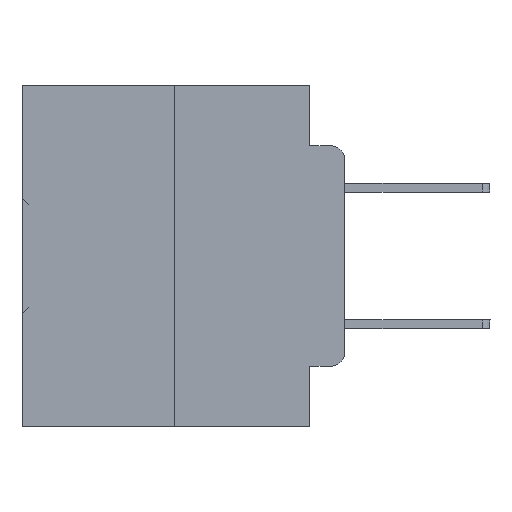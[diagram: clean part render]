
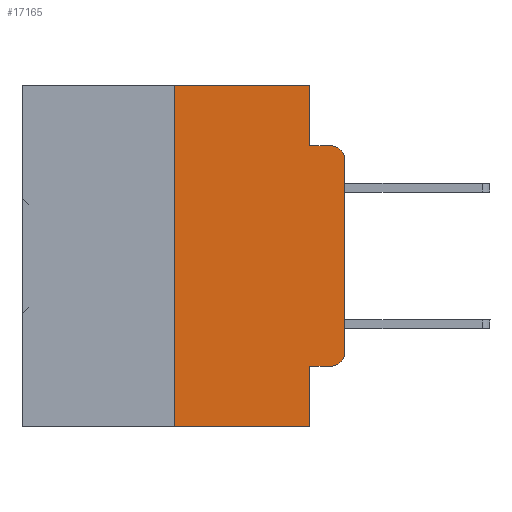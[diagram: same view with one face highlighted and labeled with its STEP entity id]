
A CAD part, left-side view. The second image highlights one B-rep face of the part: STEP entity #17165.
In plain terms, the highlighted planar face has unit normal (-1, 0, 0).
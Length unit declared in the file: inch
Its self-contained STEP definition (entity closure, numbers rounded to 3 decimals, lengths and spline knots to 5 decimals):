
#58 = EDGE_CURVE ( 'NONE', #10049, #34746, #6923, .T. ) ;
#234 = ORIENTED_EDGE ( 'NONE', *, *, #13687, .T. ) ;
#390 = CARTESIAN_POINT ( 'NONE',  ( 0., 0.473, 0. ) ) ;
#2044 = EDGE_LOOP ( 'NONE', ( #27411, #15511, #11126, #6072, #4916, #24331, #11601, #9806, #234, #10840 ) ) ;
#2606 = DIRECTION ( 'NONE',  ( 0., -1., 0. ) ) ;
#2704 = CARTESIAN_POINT ( 'NONE',  ( 0., 0.02, -0.4115 ) ) ;
#3750 = VECTOR ( 'NONE', #23329, 39.37008 ) ;
#4247 = DIRECTION ( 'NONE',  ( 0., 0., 1. ) ) ;
#4435 = EDGE_CURVE ( 'NONE', #4634, #13267, #22288, .T. ) ;
#4634 = VERTEX_POINT ( 'NONE', #22484 ) ;
#4916 = ORIENTED_EDGE ( 'NONE', *, *, #29884, .F. ) ;
#6008 = CARTESIAN_POINT ( 'NONE',  ( 0., 0.02, -0.0885 ) ) ;
#6072 = ORIENTED_EDGE ( 'NONE', *, *, #36249, .F. ) ;
#6174 = AXIS2_PLACEMENT_3D ( 'NONE', #25343, #8117, #22638 ) ;
#6923 = LINE ( 'NONE', #33304, #32812 ) ;
#8117 = DIRECTION ( 'NONE',  ( 1., 0., 0. ) ) ;
#8568 = DIRECTION ( 'NONE',  ( -1., 0., 0. ) ) ;
#8972 = DIRECTION ( 'NONE',  ( 0., 0., -1. ) ) ;
#9005 = LINE ( 'NONE', #390, #3750 ) ;
#9806 = ORIENTED_EDGE ( 'NONE', *, *, #4435, .F. ) ;
#9873 = DIRECTION ( 'NONE',  ( 0., 0., 1. ) ) ;
#10049 = VERTEX_POINT ( 'NONE', #32970 ) ;
#10840 = ORIENTED_EDGE ( 'NONE', *, *, #20039, .T. ) ;
#11126 = ORIENTED_EDGE ( 'NONE', *, *, #16709, .F. ) ;
#11536 = EDGE_CURVE ( 'NONE', #12909, #25795, #29789, .T. ) ;
#11601 = ORIENTED_EDGE ( 'NONE', *, *, #18489, .T. ) ;
#11685 = CARTESIAN_POINT ( 'NONE',  ( 0., 0.051, -0.5 ) ) ;
#11853 = CARTESIAN_POINT ( 'NONE',  ( 0., 0., -0.1085 ) ) ;
#12909 = VERTEX_POINT ( 'NONE', #31852 ) ;
#12980 = VECTOR ( 'NONE', #27152, 39.37008 ) ;
#13267 = VERTEX_POINT ( 'NONE', #11685 ) ;
#13687 = EDGE_CURVE ( 'NONE', #4634, #21027, #20557, .T. ) ;
#14054 = PLANE ( 'NONE',  #6174 ) ;
#15105 = CARTESIAN_POINT ( 'NONE',  ( 0., 0.473, -0.5 ) ) ;
#15511 = ORIENTED_EDGE ( 'NONE', *, *, #16609, .T. ) ;
#16229 = VECTOR ( 'NONE', #8972, 39.37008 ) ;
#16367 = DIRECTION ( 'NONE',  ( 0., 0., -1. ) ) ;
#16609 = EDGE_CURVE ( 'NONE', #25795, #22308, #25700, .T. ) ;
#16709 = EDGE_CURVE ( 'NONE', #36345, #22308, #19630, .T. ) ;
#17165 = ADVANCED_FACE ( 'NONE', ( #25149 ), #14054, .F. ) ;
#17486 = VECTOR ( 'NONE', #2606, 39.37008 ) ;
#18134 = CARTESIAN_POINT ( 'NONE',  ( 0., 0.051, 0. ) ) ;
#18489 = EDGE_CURVE ( 'NONE', #10049, #13267, #21007, .T. ) ;
#18982 = AXIS2_PLACEMENT_3D ( 'NONE', #33803, #24819, #36470 ) ;
#19630 = LINE ( 'NONE', #22310, #29960 ) ;
#19846 = CARTESIAN_POINT ( 'NONE',  ( 0., 0.25, 0. ) ) ;
#20039 = EDGE_CURVE ( 'NONE', #21027, #12909, #23960, .T. ) ;
#20339 = VERTEX_POINT ( 'NONE', #30192 ) ;
#20557 = LINE ( 'NONE', #28794, #17486 ) ;
#21007 = LINE ( 'NONE', #15105, #12980 ) ;
#21027 = VERTEX_POINT ( 'NONE', #2704 ) ;
#21909 = CARTESIAN_POINT ( 'NONE',  ( 0., 0.051, 0. ) ) ;
#22288 = LINE ( 'NONE', #21909, #33633 ) ;
#22308 = VERTEX_POINT ( 'NONE', #6008 ) ;
#22310 = CARTESIAN_POINT ( 'NONE',  ( 0., 0.051, -0.0885 ) ) ;
#22484 = CARTESIAN_POINT ( 'NONE',  ( 0., 0.051, -0.4115 ) ) ;
#22638 = DIRECTION ( 'NONE',  ( 0., 0., -1. ) ) ;
#23329 = DIRECTION ( 'NONE',  ( 0., -1., 0. ) ) ;
#23960 = CIRCLE ( 'NONE', #26433, 0.02 ) ;
#24331 = ORIENTED_EDGE ( 'NONE', *, *, #58, .F. ) ;
#24598 = CARTESIAN_POINT ( 'NONE',  ( 0., 0., 0. ) ) ;
#24819 = DIRECTION ( 'NONE',  ( -1., 0., 0. ) ) ;
#25149 = FACE_OUTER_BOUND ( 'NONE', #2044, .T. ) ;
#25343 = CARTESIAN_POINT ( 'NONE',  ( 0., 0.473, 0. ) ) ;
#25584 = DIRECTION ( 'NONE',  ( 0., -1., 0. ) ) ;
#25700 = CIRCLE ( 'NONE', #18982, 0.02 ) ;
#25795 = VERTEX_POINT ( 'NONE', #11853 ) ;
#26358 = CARTESIAN_POINT ( 'NONE',  ( 0., 0.02, -0.3915 ) ) ;
#26433 = AXIS2_PLACEMENT_3D ( 'NONE', #26358, #8568, #32297 ) ;
#27152 = DIRECTION ( 'NONE',  ( 0., -1., 0. ) ) ;
#27411 = ORIENTED_EDGE ( 'NONE', *, *, #11536, .T. ) ;
#28461 = VECTOR ( 'NONE', #9873, 39.37008 ) ;
#28794 = CARTESIAN_POINT ( 'NONE',  ( 0., 0.051, -0.4115 ) ) ;
#29789 = LINE ( 'NONE', #24598, #28461 ) ;
#29884 = EDGE_CURVE ( 'NONE', #34746, #20339, #9005, .T. ) ;
#29960 = VECTOR ( 'NONE', #25584, 39.37008 ) ;
#30192 = CARTESIAN_POINT ( 'NONE',  ( 0., 0.051, 0. ) ) ;
#31852 = CARTESIAN_POINT ( 'NONE',  ( 0., 0., -0.3915 ) ) ;
#32297 = DIRECTION ( 'NONE',  ( 0., 0., -1. ) ) ;
#32812 = VECTOR ( 'NONE', #4247, 39.37008 ) ;
#32872 = LINE ( 'NONE', #18134, #16229 ) ;
#32970 = CARTESIAN_POINT ( 'NONE',  ( 0., 0.25, -0.5 ) ) ;
#33058 = CARTESIAN_POINT ( 'NONE',  ( 0., 0.051, -0.0885 ) ) ;
#33304 = CARTESIAN_POINT ( 'NONE',  ( 0., 0.25, 0. ) ) ;
#33633 = VECTOR ( 'NONE', #16367, 39.37008 ) ;
#33803 = CARTESIAN_POINT ( 'NONE',  ( 0., 0.02, -0.1085 ) ) ;
#34746 = VERTEX_POINT ( 'NONE', #19846 ) ;
#36249 = EDGE_CURVE ( 'NONE', #20339, #36345, #32872, .T. ) ;
#36345 = VERTEX_POINT ( 'NONE', #33058 ) ;
#36470 = DIRECTION ( 'NONE',  ( 0., 0., -1. ) ) ;
